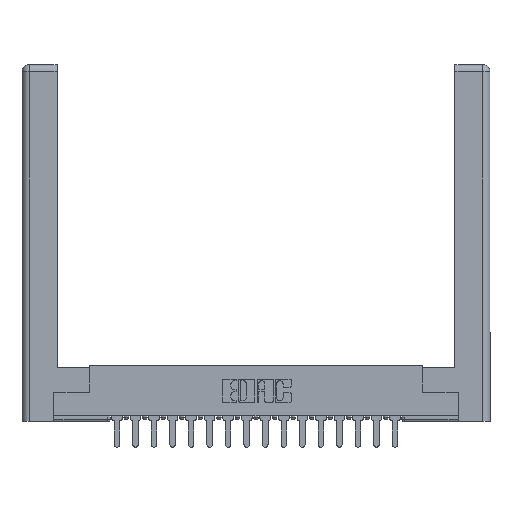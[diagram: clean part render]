
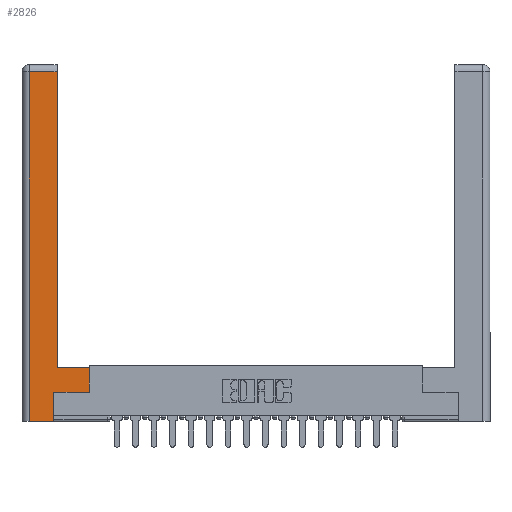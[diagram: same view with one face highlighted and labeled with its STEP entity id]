
A CAD part, top view. The second image highlights one B-rep face of the part: STEP entity #2826.
In plain terms, the highlighted planar face has unit normal (0, 0, 1).
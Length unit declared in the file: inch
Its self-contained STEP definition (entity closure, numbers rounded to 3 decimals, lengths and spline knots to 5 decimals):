
#233 = CARTESIAN_POINT ( 'NONE',  ( 0.0615, 0., 0. ) ) ;
#344 = LINE ( 'NONE', #233, #2675 ) ;
#461 = EDGE_CURVE ( 'NONE', #19774, #17838, #5243, .T. ) ;
#1433 = DIRECTION ( 'NONE',  ( -1., 0., 0. ) ) ;
#2283 = CARTESIAN_POINT ( 'NONE',  ( 0.295, 0.45, 0. ) ) ;
#2642 = CARTESIAN_POINT ( 'NONE',  ( 0.0615, 2.94, 0. ) ) ;
#2675 = VECTOR ( 'NONE', #6528, 39.37008 ) ;
#2826 = ADVANCED_FACE ( 'NONE', ( #4758 ), #7587, .F. ) ;
#2990 = EDGE_CURVE ( 'NONE', #12530, #14162, #15825, .T. ) ;
#3795 = CARTESIAN_POINT ( 'NONE',  ( 0.0615, 2.94, 0. ) ) ;
#4343 = CARTESIAN_POINT ( 'NONE',  ( 0.565, 0.245, 0. ) ) ;
#4420 = LINE ( 'NONE', #13773, #13907 ) ;
#4641 = EDGE_CURVE ( 'NONE', #14436, #19774, #4420, .T. ) ;
#4758 = FACE_OUTER_BOUND ( 'NONE', #13876, .T. ) ;
#5145 = ORIENTED_EDGE ( 'NONE', *, *, #11108, .T. ) ;
#5243 = LINE ( 'NONE', #12657, #16571 ) ;
#5346 = ORIENTED_EDGE ( 'NONE', *, *, #4641, .T. ) ;
#5367 = LINE ( 'NONE', #11547, #17778 ) ;
#5935 = AXIS2_PLACEMENT_3D ( 'NONE', #16643, #13793, #12383 ) ;
#6077 = VECTOR ( 'NONE', #1433, 39.37008 ) ;
#6161 = ORIENTED_EDGE ( 'NONE', *, *, #13478, .T. ) ;
#6512 = ORIENTED_EDGE ( 'NONE', *, *, #2990, .T. ) ;
#6528 = DIRECTION ( 'NONE',  ( 0., -1., 0. ) ) ;
#6700 = CARTESIAN_POINT ( 'NONE',  ( 0.0615, 0., 0. ) ) ;
#6742 = VECTOR ( 'NONE', #9580, 39.37008 ) ;
#6746 = LINE ( 'NONE', #19140, #6742 ) ;
#6957 = LINE ( 'NONE', #2283, #14040 ) ;
#7224 = CARTESIAN_POINT ( 'NONE',  ( 0.565, 0.45, 0. ) ) ;
#7299 = CARTESIAN_POINT ( 'NONE',  ( 0.265, 0., 0. ) ) ;
#7587 = PLANE ( 'NONE',  #5935 ) ;
#8247 = DIRECTION ( 'NONE',  ( 1., 0., 0. ) ) ;
#8715 = CARTESIAN_POINT ( 'NONE',  ( 0.295, 0.45, 0. ) ) ;
#8872 = ORIENTED_EDGE ( 'NONE', *, *, #461, .T. ) ;
#9580 = DIRECTION ( 'NONE',  ( 0., 1., 0. ) ) ;
#9992 = DIRECTION ( 'NONE',  ( 1., 0., 0. ) ) ;
#10875 = CARTESIAN_POINT ( 'NONE',  ( 0.295, 2.94, 0. ) ) ;
#11108 = EDGE_CURVE ( 'NONE', #17838, #13956, #6746, .T. ) ;
#11547 = CARTESIAN_POINT ( 'NONE',  ( 0.265, 0., 0. ) ) ;
#11629 = DIRECTION ( 'NONE',  ( -1., 0., 0. ) ) ;
#11739 = ORIENTED_EDGE ( 'NONE', *, *, #12616, .T. ) ;
#12383 = DIRECTION ( 'NONE',  ( -1., 0., 0. ) ) ;
#12431 = VECTOR ( 'NONE', #12797, 39.37008 ) ;
#12530 = VERTEX_POINT ( 'NONE', #8715 ) ;
#12616 = EDGE_CURVE ( 'NONE', #14162, #19844, #13599, .T. ) ;
#12657 = CARTESIAN_POINT ( 'NONE',  ( 0.565, 0.245, 0. ) ) ;
#12797 = DIRECTION ( 'NONE',  ( 0., 1., 0. ) ) ;
#12799 = VERTEX_POINT ( 'NONE', #6700 ) ;
#13478 = EDGE_CURVE ( 'NONE', #12799, #14436, #5367, .T. ) ;
#13528 = ORIENTED_EDGE ( 'NONE', *, *, #19771, .T. ) ;
#13599 = LINE ( 'NONE', #2642, #6077 ) ;
#13773 = CARTESIAN_POINT ( 'NONE',  ( 0.265, 0.245, 0. ) ) ;
#13789 = ORIENTED_EDGE ( 'NONE', *, *, #17624, .T. ) ;
#13793 = DIRECTION ( 'NONE',  ( 0., 0., -1. ) ) ;
#13876 = EDGE_LOOP ( 'NONE', ( #6512, #11739, #13789, #6161, #5346, #8872, #5145, #13528 ) ) ;
#13907 = VECTOR ( 'NONE', #13968, 39.37008 ) ;
#13956 = VERTEX_POINT ( 'NONE', #7224 ) ;
#13968 = DIRECTION ( 'NONE',  ( 0., 1., 0. ) ) ;
#14040 = VECTOR ( 'NONE', #11629, 39.37008 ) ;
#14162 = VERTEX_POINT ( 'NONE', #10875 ) ;
#14436 = VERTEX_POINT ( 'NONE', #7299 ) ;
#14682 = CARTESIAN_POINT ( 'NONE',  ( 0.265, 0.245, 0. ) ) ;
#15723 = CARTESIAN_POINT ( 'NONE',  ( 0.295, 3., 0. ) ) ;
#15825 = LINE ( 'NONE', #15723, #12431 ) ;
#16571 = VECTOR ( 'NONE', #8247, 39.37008 ) ;
#16643 = CARTESIAN_POINT ( 'NONE',  ( 0., 0., 0. ) ) ;
#17624 = EDGE_CURVE ( 'NONE', #19844, #12799, #344, .T. ) ;
#17778 = VECTOR ( 'NONE', #9992, 39.37008 ) ;
#17838 = VERTEX_POINT ( 'NONE', #4343 ) ;
#19140 = CARTESIAN_POINT ( 'NONE',  ( 0.565, 0.45, 0. ) ) ;
#19771 = EDGE_CURVE ( 'NONE', #13956, #12530, #6957, .T. ) ;
#19774 = VERTEX_POINT ( 'NONE', #14682 ) ;
#19844 = VERTEX_POINT ( 'NONE', #3795 ) ;
